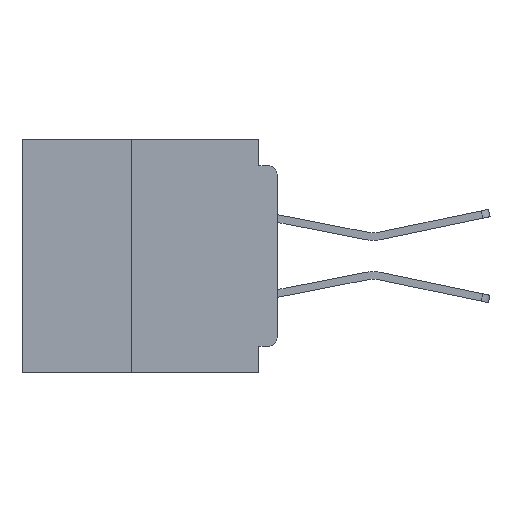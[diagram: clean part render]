
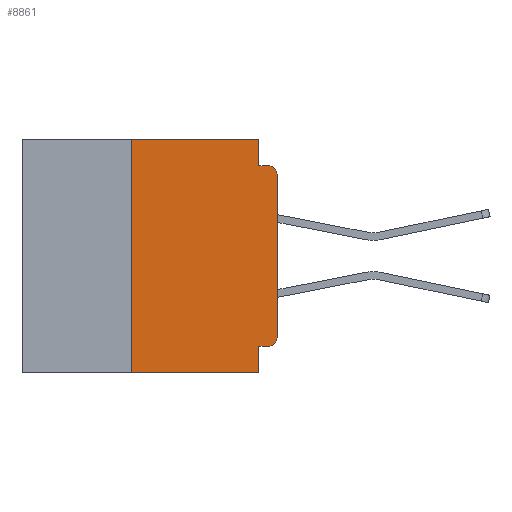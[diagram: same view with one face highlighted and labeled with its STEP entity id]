
A CAD part, left-side view. The second image highlights one B-rep face of the part: STEP entity #8861.
In plain terms, the highlighted planar face has unit normal (-1, 0, 0).
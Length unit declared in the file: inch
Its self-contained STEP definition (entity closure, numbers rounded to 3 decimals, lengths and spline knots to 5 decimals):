
#556 = ORIENTED_EDGE ( 'NONE', *, *, #34967, .T. ) ;
#741 = EDGE_CURVE ( 'NONE', #3379, #31028, #24897, .T. ) ;
#793 = DIRECTION ( 'NONE',  ( 0., 0., -1. ) ) ;
#2516 = DIRECTION ( 'NONE',  ( -1., 0., 0. ) ) ;
#2762 = DIRECTION ( 'NONE',  ( 0., 0., 1. ) ) ;
#2828 = CARTESIAN_POINT ( 'NONE',  ( 0., 0.437, 0. ) ) ;
#2891 = CARTESIAN_POINT ( 'NONE',  ( 0., 0., -0.06 ) ) ;
#3379 = VERTEX_POINT ( 'NONE', #9019 ) ;
#3824 = DIRECTION ( 'NONE',  ( 0., -1., 0. ) ) ;
#3843 = CARTESIAN_POINT ( 'NONE',  ( 0., 0.031, -0.4 ) ) ;
#4093 = ORIENTED_EDGE ( 'NONE', *, *, #19336, .T. ) ;
#6241 = DIRECTION ( 'NONE',  ( 0., 0., 1. ) ) ;
#7695 = AXIS2_PLACEMENT_3D ( 'NONE', #29998, #13340, #32811 ) ;
#8147 = VECTOR ( 'NONE', #793, 39.37008 ) ;
#8237 = ORIENTED_EDGE ( 'NONE', *, *, #10889, .F. ) ;
#8552 = PLANE ( 'NONE',  #19459 ) ;
#8861 = ADVANCED_FACE ( 'NONE', ( #22799 ), #8552, .F. ) ;
#8884 = AXIS2_PLACEMENT_3D ( 'NONE', #19381, #2516, #22163 ) ;
#9019 = CARTESIAN_POINT ( 'NONE',  ( 0., 0.25, 0. ) ) ;
#9260 = CARTESIAN_POINT ( 'NONE',  ( 0., 0.25, -0.4 ) ) ;
#9682 = CARTESIAN_POINT ( 'NONE',  ( 0., 0.031, 0. ) ) ;
#9738 = ORIENTED_EDGE ( 'NONE', *, *, #19794, .T. ) ;
#10339 = VECTOR ( 'NONE', #22646, 39.37008 ) ;
#10579 = VERTEX_POINT ( 'NONE', #2891 ) ;
#10889 = EDGE_CURVE ( 'NONE', #31028, #31074, #13592, .T. ) ;
#11274 = CARTESIAN_POINT ( 'NONE',  ( 0., 0.437, 0. ) ) ;
#11405 = DIRECTION ( 'NONE',  ( 0., 0., -1. ) ) ;
#11463 = CARTESIAN_POINT ( 'NONE',  ( 0., 0., -0.045 ) ) ;
#12725 = CARTESIAN_POINT ( 'NONE',  ( 0., 0.015, -0.045 ) ) ;
#13064 = ORIENTED_EDGE ( 'NONE', *, *, #28252, .F. ) ;
#13340 = DIRECTION ( 'NONE',  ( -1., 0., 0. ) ) ;
#13592 = LINE ( 'NONE', #9682, #27513 ) ;
#14208 = EDGE_CURVE ( 'NONE', #30318, #22196, #30409, .T. ) ;
#14308 = LINE ( 'NONE', #19625, #15167 ) ;
#14855 = ORIENTED_EDGE ( 'NONE', *, *, #23997, .F. ) ;
#15095 = CARTESIAN_POINT ( 'NONE',  ( 0., 0., -0.34 ) ) ;
#15167 = VECTOR ( 'NONE', #2762, 39.37008 ) ;
#15370 = EDGE_CURVE ( 'NONE', #35027, #3379, #19900, .T. ) ;
#15853 = CARTESIAN_POINT ( 'NONE',  ( 0., 0.437, -0.4 ) ) ;
#16160 = VERTEX_POINT ( 'NONE', #15095 ) ;
#16357 = LINE ( 'NONE', #15853, #22823 ) ;
#16867 = CARTESIAN_POINT ( 'NONE',  ( 0., 0.031, -0.4 ) ) ;
#17532 = VECTOR ( 'NONE', #3824, 39.37008 ) ;
#17897 = ORIENTED_EDGE ( 'NONE', *, *, #741, .F. ) ;
#19013 = EDGE_LOOP ( 'NONE', ( #556, #33533, #13064, #8237, #17897, #20714, #9738, #31240, #14855, #4093 ) ) ;
#19058 = CARTESIAN_POINT ( 'NONE',  ( 0., 0.031, -0.355 ) ) ;
#19336 = EDGE_CURVE ( 'NONE', #34681, #16160, #32257, .T. ) ;
#19381 = CARTESIAN_POINT ( 'NONE',  ( 0., 0.015, -0.34 ) ) ;
#19459 = AXIS2_PLACEMENT_3D ( 'NONE', #11274, #28099, #11405 ) ;
#19625 = CARTESIAN_POINT ( 'NONE',  ( 0., 0., 0. ) ) ;
#19794 = EDGE_CURVE ( 'NONE', #35027, #22196, #16357, .T. ) ;
#19900 = LINE ( 'NONE', #31396, #27284 ) ;
#20714 = ORIENTED_EDGE ( 'NONE', *, *, #15370, .F. ) ;
#21215 = CARTESIAN_POINT ( 'NONE',  ( 0., 0.015, -0.355 ) ) ;
#21969 = CIRCLE ( 'NONE', #7695, 0.015 ) ;
#22163 = DIRECTION ( 'NONE',  ( 0., 0., -1. ) ) ;
#22196 = VERTEX_POINT ( 'NONE', #16867 ) ;
#22646 = DIRECTION ( 'NONE',  ( 0., -1., 0. ) ) ;
#22799 = FACE_OUTER_BOUND ( 'NONE', #19013, .T. ) ;
#22823 = VECTOR ( 'NONE', #35251, 39.37008 ) ;
#23997 = EDGE_CURVE ( 'NONE', #34681, #30318, #35158, .T. ) ;
#24234 = VERTEX_POINT ( 'NONE', #12725 ) ;
#24897 = LINE ( 'NONE', #2828, #17532 ) ;
#24948 = CARTESIAN_POINT ( 'NONE',  ( 0., 0.031, 0. ) ) ;
#25141 = CARTESIAN_POINT ( 'NONE',  ( 0., 0., -0.355 ) ) ;
#25165 = VECTOR ( 'NONE', #27957, 39.37008 ) ;
#27284 = VECTOR ( 'NONE', #6241, 39.37008 ) ;
#27513 = VECTOR ( 'NONE', #31994, 39.37008 ) ;
#27957 = DIRECTION ( 'NONE',  ( 0., 1., 0. ) ) ;
#28016 = CARTESIAN_POINT ( 'NONE',  ( 0., 0.031, -0.045 ) ) ;
#28099 = DIRECTION ( 'NONE',  ( 1., 0., 0. ) ) ;
#28252 = EDGE_CURVE ( 'NONE', #31074, #24234, #32608, .T. ) ;
#29998 = CARTESIAN_POINT ( 'NONE',  ( 0., 0.015, -0.06 ) ) ;
#30282 = EDGE_CURVE ( 'NONE', #10579, #24234, #21969, .T. ) ;
#30318 = VERTEX_POINT ( 'NONE', #19058 ) ;
#30409 = LINE ( 'NONE', #3843, #8147 ) ;
#31028 = VERTEX_POINT ( 'NONE', #24948 ) ;
#31074 = VERTEX_POINT ( 'NONE', #28016 ) ;
#31240 = ORIENTED_EDGE ( 'NONE', *, *, #14208, .F. ) ;
#31396 = CARTESIAN_POINT ( 'NONE',  ( 0., 0.25, -0.4 ) ) ;
#31994 = DIRECTION ( 'NONE',  ( 0., 0., -1. ) ) ;
#32257 = CIRCLE ( 'NONE', #8884, 0.015 ) ;
#32608 = LINE ( 'NONE', #11463, #10339 ) ;
#32811 = DIRECTION ( 'NONE',  ( 0., 0., -1. ) ) ;
#33533 = ORIENTED_EDGE ( 'NONE', *, *, #30282, .T. ) ;
#34681 = VERTEX_POINT ( 'NONE', #21215 ) ;
#34967 = EDGE_CURVE ( 'NONE', #16160, #10579, #14308, .T. ) ;
#35027 = VERTEX_POINT ( 'NONE', #9260 ) ;
#35158 = LINE ( 'NONE', #25141, #25165 ) ;
#35251 = DIRECTION ( 'NONE',  ( 0., -1., 0. ) ) ;
